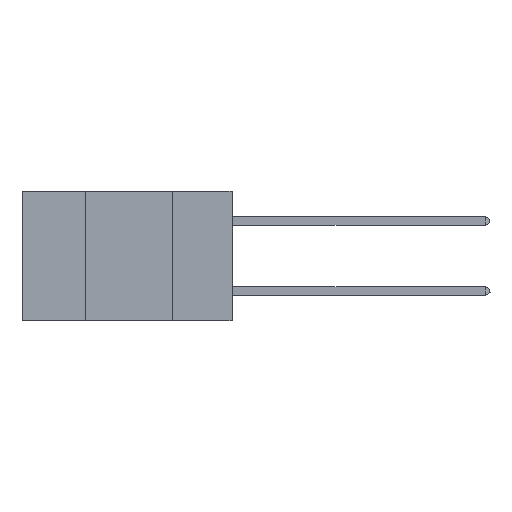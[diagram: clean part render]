
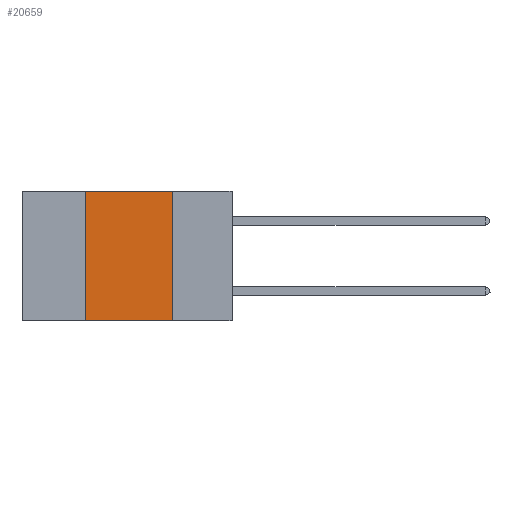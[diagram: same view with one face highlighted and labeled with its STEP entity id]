
A CAD part, left-side view. The second image highlights one B-rep face of the part: STEP entity #20659.
In plain terms, the highlighted planar face has unit normal (-1, 0, 0).
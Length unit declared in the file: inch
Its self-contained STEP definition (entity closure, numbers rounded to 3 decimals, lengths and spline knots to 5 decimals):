
#340 = LINE ( 'NONE', #14330, #5196 ) ;
#893 = VECTOR ( 'NONE', #6310, 39.37008 ) ;
#1257 = VERTEX_POINT ( 'NONE', #3440 ) ;
#3440 = CARTESIAN_POINT ( 'NONE',  ( 0., 0.42, -0.37 ) ) ;
#3669 = CARTESIAN_POINT ( 'NONE',  ( 0., 0.6, -0.37 ) ) ;
#4248 = EDGE_CURVE ( 'NONE', #12917, #21376, #340, .T. ) ;
#4506 = FACE_OUTER_BOUND ( 'NONE', #29531, .T. ) ;
#4988 = CARTESIAN_POINT ( 'NONE',  ( 0., 0.17, -0.37 ) ) ;
#5196 = VECTOR ( 'NONE', #14099, 39.37008 ) ;
#5592 = AXIS2_PLACEMENT_3D ( 'NONE', #18031, #28746, #31542 ) ;
#6310 = DIRECTION ( 'NONE',  ( 0., 0., -1. ) ) ;
#6772 = CARTESIAN_POINT ( 'NONE',  ( 0., 0.42, 0. ) ) ;
#7325 = CARTESIAN_POINT ( 'NONE',  ( 0., 0.42, 0. ) ) ;
#7539 = VERTEX_POINT ( 'NONE', #4988 ) ;
#7546 = LINE ( 'NONE', #3669, #34977 ) ;
#8869 = EDGE_CURVE ( 'NONE', #21376, #7539, #35799, .T. ) ;
#9401 = PLANE ( 'NONE',  #5592 ) ;
#9496 = DIRECTION ( 'NONE',  ( 0., -1., 0. ) ) ;
#12869 = EDGE_CURVE ( 'NONE', #1257, #12917, #20212, .T. ) ;
#12917 = VERTEX_POINT ( 'NONE', #7325 ) ;
#14099 = DIRECTION ( 'NONE',  ( 0., -1., 0. ) ) ;
#14330 = CARTESIAN_POINT ( 'NONE',  ( 0., 0.6, 0. ) ) ;
#14723 = ORIENTED_EDGE ( 'NONE', *, *, #4248, .F. ) ;
#18012 = CARTESIAN_POINT ( 'NONE',  ( 0., 0.17, 0. ) ) ;
#18031 = CARTESIAN_POINT ( 'NONE',  ( 0., 0.6, 0. ) ) ;
#20212 = LINE ( 'NONE', #6772, #23259 ) ;
#20456 = DIRECTION ( 'NONE',  ( 0., 0., 1. ) ) ;
#20659 = ADVANCED_FACE ( 'NONE', ( #4506 ), #9401, .F. ) ;
#21376 = VERTEX_POINT ( 'NONE', #18012 ) ;
#23259 = VECTOR ( 'NONE', #20456, 39.37008 ) ;
#23456 = ORIENTED_EDGE ( 'NONE', *, *, #8869, .F. ) ;
#28682 = CARTESIAN_POINT ( 'NONE',  ( 0., 0.17, 0. ) ) ;
#28746 = DIRECTION ( 'NONE',  ( 1., 0., 0. ) ) ;
#29531 = EDGE_LOOP ( 'NONE', ( #23456, #14723, #34413, #31983 ) ) ;
#31542 = DIRECTION ( 'NONE',  ( 0., 0., -1. ) ) ;
#31621 = EDGE_CURVE ( 'NONE', #1257, #7539, #7546, .T. ) ;
#31983 = ORIENTED_EDGE ( 'NONE', *, *, #31621, .T. ) ;
#34413 = ORIENTED_EDGE ( 'NONE', *, *, #12869, .F. ) ;
#34977 = VECTOR ( 'NONE', #9496, 39.37008 ) ;
#35799 = LINE ( 'NONE', #28682, #893 ) ;
